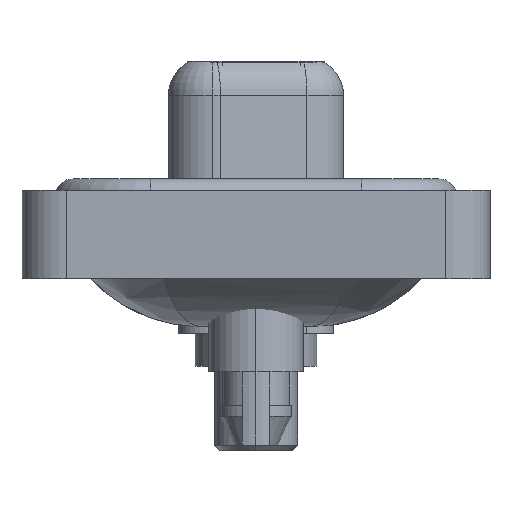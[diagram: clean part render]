
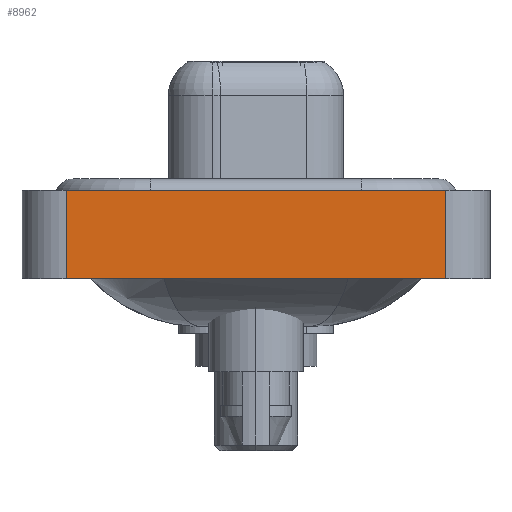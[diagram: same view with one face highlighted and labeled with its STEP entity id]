
A CAD part, left-side view. The second image highlights one B-rep face of the part: STEP entity #8962.
In plain terms, the highlighted planar face has unit normal (-1, 0, 0).
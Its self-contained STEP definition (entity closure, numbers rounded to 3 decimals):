
#48 = PLANE ( 'NONE',  #1371 ) ;
#66 = EDGE_CURVE ( 'NONE', #15747, #5555, #14625, .T. ) ;
#1371 = AXIS2_PLACEMENT_3D ( 'NONE', #2386, #10658, #16134 ) ;
#1512 = CARTESIAN_POINT ( 'NONE',  ( -7.3, 8.55, 0.4 ) ) ;
#2318 = CARTESIAN_POINT ( 'NONE',  ( -7.3, -8.55, 0.4 ) ) ;
#2386 = CARTESIAN_POINT ( 'NONE',  ( -7.3, -8.55, -3.6 ) ) ;
#2459 = LINE ( 'NONE', #13048, #13900 ) ;
#3017 = EDGE_CURVE ( 'NONE', #5343, #5555, #13260, .T. ) ;
#3682 = CARTESIAN_POINT ( 'NONE',  ( -7.3, -8.55, -3.6 ) ) ;
#5343 = VERTEX_POINT ( 'NONE', #12169 ) ;
#5555 = VERTEX_POINT ( 'NONE', #2318 ) ;
#6450 = EDGE_CURVE ( 'NONE', #11894, #15747, #14926, .T. ) ;
#7858 = DIRECTION ( 'NONE',  ( 0., -1., 0. ) ) ;
#8151 = ORIENTED_EDGE ( 'NONE', *, *, #6450, .F. ) ;
#8263 = CARTESIAN_POINT ( 'NONE',  ( -7.3, 8.55, -3.6 ) ) ;
#8852 = VECTOR ( 'NONE', #14965, 1000. ) ;
#8962 = ADVANCED_FACE ( 'NONE', ( #13473 ), #48, .T. ) ;
#10545 = VECTOR ( 'NONE', #12936, 1000. ) ;
#10658 = DIRECTION ( 'NONE',  ( -1., 0., 0. ) ) ;
#11215 = DIRECTION ( 'NONE',  ( 0., 0., 1. ) ) ;
#11434 = VECTOR ( 'NONE', #11215, 1000. ) ;
#11894 = VERTEX_POINT ( 'NONE', #15756 ) ;
#12169 = CARTESIAN_POINT ( 'NONE',  ( -7.3, -8.55, -3.6 ) ) ;
#12387 = ORIENTED_EDGE ( 'NONE', *, *, #3017, .T. ) ;
#12936 = DIRECTION ( 'NONE',  ( 0., 0., 1. ) ) ;
#13048 = CARTESIAN_POINT ( 'NONE',  ( -7.3, -8.55, -3.6 ) ) ;
#13260 = LINE ( 'NONE', #3682, #10545 ) ;
#13473 = FACE_OUTER_BOUND ( 'NONE', #14115, .T. ) ;
#13900 = VECTOR ( 'NONE', #7858, 1000. ) ;
#14115 = EDGE_LOOP ( 'NONE', ( #12387, #15201, #8151, #16641 ) ) ;
#14625 = LINE ( 'NONE', #17544, #8852 ) ;
#14926 = LINE ( 'NONE', #8263, #11434 ) ;
#14965 = DIRECTION ( 'NONE',  ( 0., -1., 0. ) ) ;
#15201 = ORIENTED_EDGE ( 'NONE', *, *, #66, .F. ) ;
#15747 = VERTEX_POINT ( 'NONE', #1512 ) ;
#15756 = CARTESIAN_POINT ( 'NONE',  ( -7.3, 8.55, -3.6 ) ) ;
#16100 = EDGE_CURVE ( 'NONE', #11894, #5343, #2459, .T. ) ;
#16134 = DIRECTION ( 'NONE',  ( 0., 0., 1. ) ) ;
#16641 = ORIENTED_EDGE ( 'NONE', *, *, #16100, .T. ) ;
#17544 = CARTESIAN_POINT ( 'NONE',  ( -7.3, -8.55, 0.4 ) ) ;
